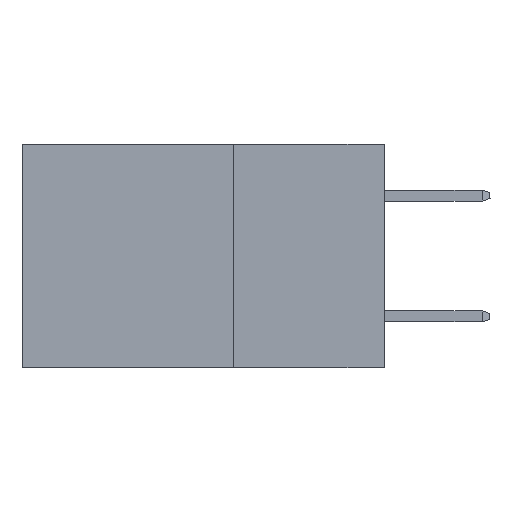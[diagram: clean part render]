
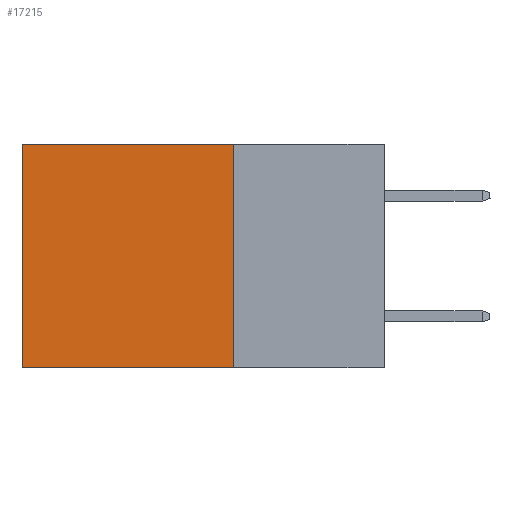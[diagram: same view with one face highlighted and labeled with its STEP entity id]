
A CAD part, left-side view. The second image highlights one B-rep face of the part: STEP entity #17215.
In plain terms, the highlighted planar face has unit normal (-1, 0, 0).
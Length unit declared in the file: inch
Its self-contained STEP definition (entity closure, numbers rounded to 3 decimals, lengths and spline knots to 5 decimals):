
#672 = EDGE_CURVE ( 'NONE', #5787, #17181, #17544, .T. ) ;
#2800 = CARTESIAN_POINT ( 'NONE',  ( 0.298, 0.6, 0. ) ) ;
#2805 = CARTESIAN_POINT ( 'NONE',  ( 0.298, 0.25, 0. ) ) ;
#4907 = DIRECTION ( 'NONE',  ( 0., 0., -1. ) ) ;
#5787 = VERTEX_POINT ( 'NONE', #21210 ) ;
#5817 = VECTOR ( 'NONE', #9114, 39.37008 ) ;
#7746 = VERTEX_POINT ( 'NONE', #13159 ) ;
#8941 = CARTESIAN_POINT ( 'NONE',  ( 0.298, 0.25, 0. ) ) ;
#9018 = CARTESIAN_POINT ( 'NONE',  ( 0.298, 0.6, 0. ) ) ;
#9114 = DIRECTION ( 'NONE',  ( 0., 0., -1. ) ) ;
#9144 = VERTEX_POINT ( 'NONE', #2800 ) ;
#10715 = LINE ( 'NONE', #9018, #16156 ) ;
#10782 = EDGE_CURVE ( 'NONE', #7746, #9144, #13078, .T. ) ;
#11047 = EDGE_CURVE ( 'NONE', #9144, #17181, #10715, .T. ) ;
#11051 = DIRECTION ( 'NONE',  ( 1., 0., 0. ) ) ;
#12484 = DIRECTION ( 'NONE',  ( 0., 1., 0. ) ) ;
#12622 = ORIENTED_EDGE ( 'NONE', *, *, #24756, .F. ) ;
#13078 = LINE ( 'NONE', #26735, #13731 ) ;
#13159 = CARTESIAN_POINT ( 'NONE',  ( 0.298, 0.25, 0. ) ) ;
#13731 = VECTOR ( 'NONE', #14386, 39.37008 ) ;
#14386 = DIRECTION ( 'NONE',  ( 0., 1., 0. ) ) ;
#15611 = ORIENTED_EDGE ( 'NONE', *, *, #10782, .T. ) ;
#16156 = VECTOR ( 'NONE', #4907, 39.37008 ) ;
#16670 = ORIENTED_EDGE ( 'NONE', *, *, #672, .F. ) ;
#16815 = LINE ( 'NONE', #2805, #5817 ) ;
#17056 = CARTESIAN_POINT ( 'NONE',  ( 0.298, 0.6, -0.37 ) ) ;
#17181 = VERTEX_POINT ( 'NONE', #17056 ) ;
#17215 = ADVANCED_FACE ( 'NONE', ( #24216 ), #21263, .F. ) ;
#17544 = LINE ( 'NONE', #25945, #22421 ) ;
#19159 = EDGE_LOOP ( 'NONE', ( #26814, #16670, #12622, #15611 ) ) ;
#21210 = CARTESIAN_POINT ( 'NONE',  ( 0.298, 0.25, -0.37 ) ) ;
#21263 = PLANE ( 'NONE',  #22863 ) ;
#22421 = VECTOR ( 'NONE', #12484, 39.37008 ) ;
#22863 = AXIS2_PLACEMENT_3D ( 'NONE', #8941, #11051, #25436 ) ;
#24216 = FACE_OUTER_BOUND ( 'NONE', #19159, .T. ) ;
#24756 = EDGE_CURVE ( 'NONE', #7746, #5787, #16815, .T. ) ;
#25436 = DIRECTION ( 'NONE',  ( 0., 0., -1. ) ) ;
#25945 = CARTESIAN_POINT ( 'NONE',  ( 0.298, 0.25, -0.37 ) ) ;
#26735 = CARTESIAN_POINT ( 'NONE',  ( 0.298, 0.25, 0. ) ) ;
#26814 = ORIENTED_EDGE ( 'NONE', *, *, #11047, .T. ) ;
